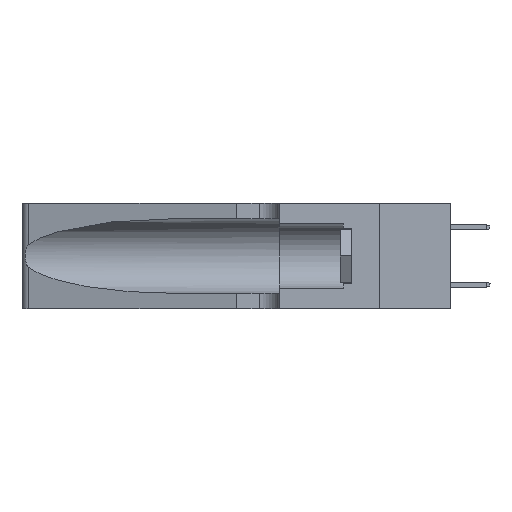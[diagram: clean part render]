
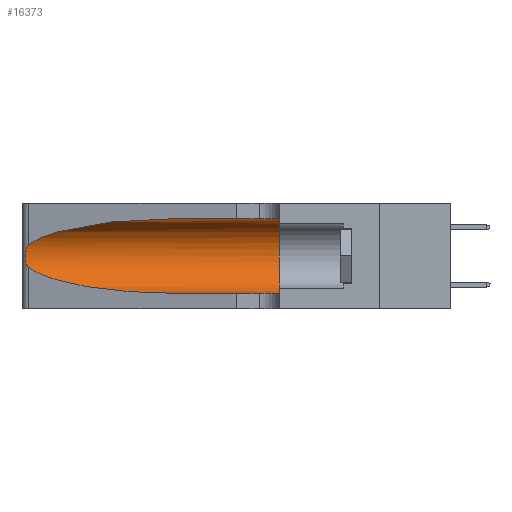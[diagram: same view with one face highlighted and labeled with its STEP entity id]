
A CAD part, left-side view. The second image highlights one B-rep face of the part: STEP entity #16373.
In plain terms, the highlighted cylindrical face has radius 3.308 mm (diameter 6.617 mm), a partial arc.
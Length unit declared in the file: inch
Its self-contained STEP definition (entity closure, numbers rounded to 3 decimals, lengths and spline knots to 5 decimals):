
#683 = CARTESIAN_POINT ( 'NONE',  ( 0.1305, 0.72297, 0.31525 ) ) ;
#1268 = VERTEX_POINT ( 'NONE', #24833 ) ;
#3240 = B_SPLINE_CURVE_WITH_KNOTS ( 'NONE', 3,
 ( #38177, #34456, #14427, #22031, #34685, #27924, #4661, #17924, #27721, #8783, #7930, #35319, #28145, #41243 ),
 .UNSPECIFIED., .F., .F.,
 ( 4, 2, 2, 2, 2, 2, 4 ),
 ( 0., 0.00027, 0.00053, 0.00107, 0.0016, 0.00187, 0.00214 ),
 .UNSPECIFIED. ) ;
#4661 = CARTESIAN_POINT ( 'NONE',  ( 0.26075, 1.23896, 0.19203 ) ) ;
#4726 = CARTESIAN_POINT ( 'NONE',  ( 0.1305, 0.72297, 0.31525 ) ) ;
#5316 = CARTESIAN_POINT ( 'NONE',  ( 0.1305, 0.72297, 0.05475 ) ) ;
#6548 = ORIENTED_EDGE ( 'NONE', *, *, #11203, .T. ) ;
#6991 = EDGE_CURVE ( 'NONE', #20251, #16871, #26199, .T. ) ;
#7423 = CARTESIAN_POINT ( 'NONE',  ( 0.25487, 1.22718, 0.22369 ) ) ;
#7724 =( BOUNDED_CURVE ( )  B_SPLINE_CURVE ( 3, ( #683, #20884, #37231, #7423 ),
 .UNSPECIFIED., .F., .T. ) 
 B_SPLINE_CURVE_WITH_KNOTS ( ( 4, 4 ),
 ( 1.5708, 2.84003 ),
 .UNSPECIFIED. ) 
 CURVE ( )  GEOMETRIC_REPRESENTATION_ITEM ( )  RATIONAL_B_SPLINE_CURVE ( ( 1., 0.87, 0.87, 1. ) ) 
 REPRESENTATION_ITEM ( '' )  );
#7930 = CARTESIAN_POINT ( 'NONE',  ( 0.25789, 1.23486, 0.15765 ) ) ;
#8232 =( BOUNDED_CURVE ( )  B_SPLINE_CURVE ( 3, ( #38398, #12483, #38196, #5316 ),
 .UNSPECIFIED., .F., .F. ) 
 B_SPLINE_CURVE_WITH_KNOTS ( ( 4, 4 ),
 ( 3.44316, 4.71239 ),
 .UNSPECIFIED. ) 
 CURVE ( )  GEOMETRIC_REPRESENTATION_ITEM ( )  RATIONAL_B_SPLINE_CURVE ( ( 1., 0.87, 0.87, 1. ) ) 
 REPRESENTATION_ITEM ( '' )  );
#8479 = CARTESIAN_POINT ( 'NONE',  ( 0.1305, 0.35, 0.05475 ) ) ;
#8577 = DIRECTION ( 'NONE',  ( 0., 0., -1. ) ) ;
#8783 = CARTESIAN_POINT ( 'NONE',  ( 0.25856, 1.23593, 0.16098 ) ) ;
#9070 = CARTESIAN_POINT ( 'NONE',  ( 0.1305, 0.72297, 0.05475 ) ) ;
#11203 = EDGE_CURVE ( 'NONE', #1268, #11781, #3240, .T. ) ;
#11781 = VERTEX_POINT ( 'NONE', #22622 ) ;
#11797 = ORIENTED_EDGE ( 'NONE', *, *, #6991, .F. ) ;
#12483 = CARTESIAN_POINT ( 'NONE',  ( 0.2373, 1.15595, 0.08982 ) ) ;
#13675 = CARTESIAN_POINT ( 'NONE',  ( 0.1305, 0.35, 0.31525 ) ) ;
#13836 = LINE ( 'NONE', #33442, #41963 ) ;
#14427 = CARTESIAN_POINT ( 'NONE',  ( 0.25639, 1.23184, 0.21858 ) ) ;
#16373 = ADVANCED_FACE ( 'NONE', ( #21186 ), #27728, .F. ) ;
#16871 = VERTEX_POINT ( 'NONE', #8479 ) ;
#17924 = CARTESIAN_POINT ( 'NONE',  ( 0.26075, 1.23896, 0.178 ) ) ;
#18557 = AXIS2_PLACEMENT_3D ( 'NONE', #25099, #28377, #8577 ) ;
#20251 = VERTEX_POINT ( 'NONE', #13675 ) ;
#20884 = CARTESIAN_POINT ( 'NONE',  ( 0.18966, 0.96281, 0.31525 ) ) ;
#21186 = FACE_OUTER_BOUND ( 'NONE', #41935, .T. ) ;
#21320 = DIRECTION ( 'NONE',  ( 0., 1., 0. ) ) ;
#21991 = AXIS2_PLACEMENT_3D ( 'NONE', #37470, #21320, #33978 ) ;
#22031 = CARTESIAN_POINT ( 'NONE',  ( 0.25787, 1.23484, 0.2124 ) ) ;
#22556 = VERTEX_POINT ( 'NONE', #9070 ) ;
#22622 = CARTESIAN_POINT ( 'NONE',  ( 0.25487, 1.22718, 0.14631 ) ) ;
#23826 = LINE ( 'NONE', #36686, #28281 ) ;
#24833 = CARTESIAN_POINT ( 'NONE',  ( 0.25487, 1.22718, 0.22369 ) ) ;
#25099 = CARTESIAN_POINT ( 'NONE',  ( 0.1305, 1.61858, 0.185 ) ) ;
#25430 = ORIENTED_EDGE ( 'NONE', *, *, #41745, .T. ) ;
#26153 = EDGE_CURVE ( 'NONE', #40132, #1268, #7724, .T. ) ;
#26199 = CIRCLE ( 'NONE', #21991, 0.13025 ) ;
#27025 = EDGE_CURVE ( 'NONE', #40132, #20251, #13836, .T. ) ;
#27119 = DIRECTION ( 'NONE',  ( 0., -1., 0. ) ) ;
#27721 = CARTESIAN_POINT ( 'NONE',  ( 0.26017, 1.23833, 0.17102 ) ) ;
#27728 = CYLINDRICAL_SURFACE ( 'NONE', #18557, 0.13025 ) ;
#27924 = CARTESIAN_POINT ( 'NONE',  ( 0.26018, 1.23835, 0.19895 ) ) ;
#28145 = CARTESIAN_POINT ( 'NONE',  ( 0.25555, 1.22993, 0.14849 ) ) ;
#28281 = VECTOR ( 'NONE', #40194, 39.37008 ) ;
#28377 = DIRECTION ( 'NONE',  ( 0., -1., 0. ) ) ;
#32577 = ORIENTED_EDGE ( 'NONE', *, *, #35369, .T. ) ;
#33442 = CARTESIAN_POINT ( 'NONE',  ( 0.1305, 1.61858, 0.31525 ) ) ;
#33978 = DIRECTION ( 'NONE',  ( 0., 0., 1. ) ) ;
#34387 = ORIENTED_EDGE ( 'NONE', *, *, #26153, .T. ) ;
#34456 = CARTESIAN_POINT ( 'NONE',  ( 0.25555, 1.22994, 0.2215 ) ) ;
#34685 = CARTESIAN_POINT ( 'NONE',  ( 0.25854, 1.2359, 0.20912 ) ) ;
#35319 = CARTESIAN_POINT ( 'NONE',  ( 0.25639, 1.23186, 0.15144 ) ) ;
#35369 = EDGE_CURVE ( 'NONE', #11781, #22556, #8232, .T. ) ;
#36686 = CARTESIAN_POINT ( 'NONE',  ( 0.1305, 1.61858, 0.05475 ) ) ;
#37231 = CARTESIAN_POINT ( 'NONE',  ( 0.2373, 1.15595, 0.28018 ) ) ;
#37470 = CARTESIAN_POINT ( 'NONE',  ( 0.1305, 0.35, 0.185 ) ) ;
#38177 = CARTESIAN_POINT ( 'NONE',  ( 0.25487, 1.22718, 0.22369 ) ) ;
#38196 = CARTESIAN_POINT ( 'NONE',  ( 0.18966, 0.96281, 0.05475 ) ) ;
#38398 = CARTESIAN_POINT ( 'NONE',  ( 0.25487, 1.22718, 0.14631 ) ) ;
#39330 = ORIENTED_EDGE ( 'NONE', *, *, #27025, .F. ) ;
#40132 = VERTEX_POINT ( 'NONE', #4726 ) ;
#40194 = DIRECTION ( 'NONE',  ( 0., -1., 0. ) ) ;
#41243 = CARTESIAN_POINT ( 'NONE',  ( 0.25487, 1.22718, 0.14631 ) ) ;
#41745 = EDGE_CURVE ( 'NONE', #22556, #16871, #23826, .T. ) ;
#41935 = EDGE_LOOP ( 'NONE', ( #34387, #6548, #32577, #25430, #11797, #39330 ) ) ;
#41963 = VECTOR ( 'NONE', #27119, 39.37008 ) ;
